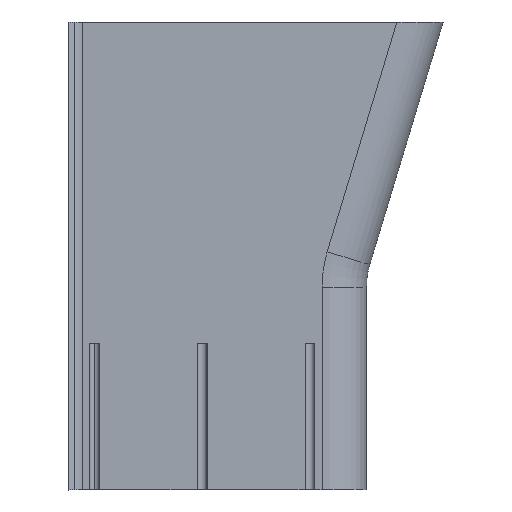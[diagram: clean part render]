
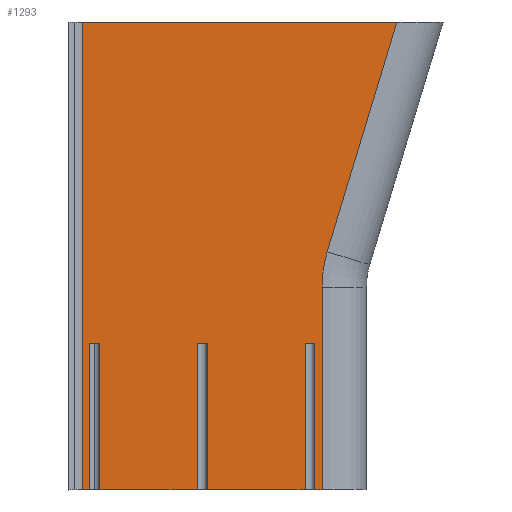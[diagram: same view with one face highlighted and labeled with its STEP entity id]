
A CAD part, left-side view. The second image highlights one B-rep face of the part: STEP entity #1293.
In plain terms, the highlighted planar face has unit normal (-1, 0, 0).
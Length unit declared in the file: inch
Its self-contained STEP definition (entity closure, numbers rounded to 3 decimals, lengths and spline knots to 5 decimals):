
#1 = VERTEX_POINT ( 'NONE', #1411 ) ;
#2 = DIRECTION ( 'NONE',  ( 0., -1., 0. ) ) ;
#8 = CARTESIAN_POINT ( 'NONE',  ( 4.52259, 2.87607, 6.34768 ) ) ;
#33 = CARTESIAN_POINT ( 'NONE',  ( 4.52259, 5.96984, 6.34768 ) ) ;
#66 = CARTESIAN_POINT ( 'NONE',  ( 4.52259, 4.9122, 1.57196 ) ) ;
#107 = VECTOR ( 'NONE', #1693, 39.37008 ) ;
#110 = VECTOR ( 'NONE', #1736, 39.37008 ) ;
#112 = LINE ( 'NONE', #1727, #110 ) ;
#113 = LINE ( 'NONE', #1715, #107 ) ;
#118 = LINE ( 'NONE', #1712, #127 ) ;
#127 = VECTOR ( 'NONE', #1710, 39.37008 ) ;
#130 = VECTOR ( 'NONE', #339, 39.37008 ) ;
#150 = VECTOR ( 'NONE', #289, 39.37008 ) ;
#156 = LINE ( 'NONE', #372, #150 ) ;
#160 = LINE ( 'NONE', #497, #130 ) ;
#168 = VECTOR ( 'NONE', #1691, 39.37008 ) ;
#169 = DIRECTION ( 'NONE',  ( 0., 1., 0. ) ) ;
#170 = VERTEX_POINT ( 'NONE', #1612 ) ;
#175 = LINE ( 'NONE', #1702, #168 ) ;
#179 = CARTESIAN_POINT ( 'NONE',  ( 4.52259, 3.63903, 1.57196 ) ) ;
#203 = LINE ( 'NONE', #685, #628 ) ;
#214 = CARTESIAN_POINT ( 'NONE',  ( 4.52259, 3.7122, 1.57196 ) ) ;
#216 = LINE ( 'NONE', #609, #410 ) ;
#231 = DIRECTION ( 'NONE',  ( 0., 1., 0. ) ) ;
#232 = CARTESIAN_POINT ( 'NONE',  ( 4.52259, 3.63903, 1.57196 ) ) ;
#237 = LINE ( 'NONE', #953, #244 ) ;
#244 = VECTOR ( 'NONE', #927, 39.37008 ) ;
#246 = DIRECTION ( 'NONE',  ( 0., 0., 1. ) ) ;
#255 = DIRECTION ( 'NONE',  ( -1., 0., 0. ) ) ;
#258 = CARTESIAN_POINT ( 'NONE',  ( 4.52259, 5.96984, 8.02732 ) ) ;
#272 = FACE_OUTER_BOUND ( 'NONE', #1458, .T. ) ;
#278 = PLANE ( 'NONE',  #649 ) ;
#289 = DIRECTION ( 'NONE',  ( 0., 0., -1. ) ) ;
#339 = DIRECTION ( 'NONE',  ( 0., 0., -1. ) ) ;
#365 = EDGE_CURVE ( 'NONE', #1374, #170, #786, .T. ) ;
#372 = CARTESIAN_POINT ( 'NONE',  ( 4.52259, 5.9122, 7.01889 ) ) ;
#410 = VECTOR ( 'NONE', #601, 39.37008 ) ;
#422 = CARTESIAN_POINT ( 'NONE',  ( 4.52259, 5.9122, 1.57196 ) ) ;
#423 = VECTOR ( 'NONE', #169, 39.37008 ) ;
#424 = LINE ( 'NONE', #179, #423 ) ;
#425 = DIRECTION ( 'NONE',  ( 0., 0., -1. ) ) ;
#427 = CARTESIAN_POINT ( 'NONE',  ( 4.52259, 4.8122, 7.01889 ) ) ;
#443 = VECTOR ( 'NONE', #1273, 39.37008 ) ;
#448 = LINE ( 'NONE', #232, #453 ) ;
#453 = VECTOR ( 'NONE', #231, 39.37008 ) ;
#490 = CARTESIAN_POINT ( 'NONE',  ( 4.52259, 6.0122, 1.57196 ) ) ;
#497 = CARTESIAN_POINT ( 'NONE',  ( 4.52259, 4.9122, 7.01889 ) ) ;
#515 = VERTEX_POINT ( 'NONE', #490 ) ;
#538 = DIRECTION ( 'NONE',  ( 0., 1., 0. ) ) ;
#539 = CARTESIAN_POINT ( 'NONE',  ( 4.52259, 3.63903, 1.57196 ) ) ;
#554 = LINE ( 'NONE', #427, #563 ) ;
#563 = VECTOR ( 'NONE', #425, 39.37008 ) ;
#570 = VERTEX_POINT ( 'NONE', #422 ) ;
#601 = DIRECTION ( 'NONE',  ( 0., 1., 0. ) ) ;
#608 = VECTOR ( 'NONE', #538, 39.37008 ) ;
#609 = CARTESIAN_POINT ( 'NONE',  ( 4.52259, 4.90544, 3.07196 ) ) ;
#610 = LINE ( 'NONE', #539, #608 ) ;
#628 = VECTOR ( 'NONE', #655, 39.37008 ) ;
#649 = AXIS2_PLACEMENT_3D ( 'NONE', #258, #255, #246 ) ;
#655 = DIRECTION ( 'NONE',  ( 0., 1., 0. ) ) ;
#668 = VECTOR ( 'NONE', #1101, 39.37008 ) ;
#673 = LINE ( 'NONE', #1129, #668 ) ;
#678 = VECTOR ( 'NONE', #1203, 39.37008 ) ;
#684 = LINE ( 'NONE', #1240, #678 ) ;
#685 = CARTESIAN_POINT ( 'NONE',  ( 4.52259, 3.63903, 1.57196 ) ) ;
#721 = DIRECTION ( 'NONE',  ( 0., 0., 1. ) ) ;
#724 = VECTOR ( 'NONE', #2, 39.37008 ) ;
#726 = EDGE_CURVE ( 'NONE', #1658, #1162, #727, .T. ) ;
#727 = LINE ( 'NONE', #33, #724 ) ;
#768 = DIRECTION ( 'NONE',  ( 1., 0., 0. ) ) ;
#786 = CIRCLE ( 'NONE', #884, 1.24053 ) ;
#805 = VERTEX_POINT ( 'NONE', #1672 ) ;
#808 = CARTESIAN_POINT ( 'NONE',  ( 4.52259, 2.3985, 3.64246 ) ) ;
#852 = VERTEX_POINT ( 'NONE', #1632 ) ;
#884 = AXIS2_PLACEMENT_3D ( 'NONE', #808, #768, #721 ) ;
#927 = DIRECTION ( 'NONE',  ( 0., 0., -1. ) ) ;
#941 = LINE ( 'NONE', #1333, #443 ) ;
#953 = CARTESIAN_POINT ( 'NONE',  ( 4.52259, 6.0122, 7.01889 ) ) ;
#989 = EDGE_CURVE ( 'NONE', #1, #1576, #684, .T. ) ;
#992 = VERTEX_POINT ( 'NONE', #1151 ) ;
#1013 = VERTEX_POINT ( 'NONE', #1133 ) ;
#1018 = EDGE_CURVE ( 'NONE', #1658, #1013, #673, .T. ) ;
#1055 = ORIENTED_EDGE ( 'NONE', *, *, #1419, .T. ) ;
#1083 = ORIENTED_EDGE ( 'NONE', *, *, #1412, .F. ) ;
#1088 = ORIENTED_EDGE ( 'NONE', *, *, #1300, .F. ) ;
#1092 = ORIENTED_EDGE ( 'NONE', *, *, #1246, .T. ) ;
#1094 = ORIENTED_EDGE ( 'NONE', *, *, #1441, .F. ) ;
#1097 = ORIENTED_EDGE ( 'NONE', *, *, #1322, .F. ) ;
#1098 = ORIENTED_EDGE ( 'NONE', *, *, #1018, .T. ) ;
#1101 = DIRECTION ( 'NONE',  ( 0., 0., -1. ) ) ;
#1126 = ORIENTED_EDGE ( 'NONE', *, *, #1706, .T. ) ;
#1129 = CARTESIAN_POINT ( 'NONE',  ( 4.52259, 6.08537, 8.02732 ) ) ;
#1133 = CARTESIAN_POINT ( 'NONE',  ( 4.52259, 6.08537, 1.57196 ) ) ;
#1151 = CARTESIAN_POINT ( 'NONE',  ( 4.52259, 6.0122, 3.07196 ) ) ;
#1161 = ORIENTED_EDGE ( 'NONE', *, *, #1400, .F. ) ;
#1162 = VERTEX_POINT ( 'NONE', #8 ) ;
#1185 = EDGE_CURVE ( 'NONE', #805, #1309, #203, .T. ) ;
#1203 = DIRECTION ( 'NONE',  ( 0., -1., 0. ) ) ;
#1223 = EDGE_CURVE ( 'NONE', #1556, #852, #610, .T. ) ;
#1240 = CARTESIAN_POINT ( 'NONE',  ( 4.52259, 4.90544, 3.07196 ) ) ;
#1246 = EDGE_CURVE ( 'NONE', #1549, #852, #554, .T. ) ;
#1273 = DIRECTION ( 'NONE',  ( 0., -1., 0. ) ) ;
#1293 = ADVANCED_FACE ( 'NONE', ( #272 ), #278, .T. ) ;
#1300 = EDGE_CURVE ( 'NONE', #1439, #570, #448, .T. ) ;
#1309 = VERTEX_POINT ( 'NONE', #214 ) ;
#1322 = EDGE_CURVE ( 'NONE', #515, #1013, #424, .T. ) ;
#1331 = ORIENTED_EDGE ( 'NONE', *, *, #1185, .F. ) ;
#1333 = CARTESIAN_POINT ( 'NONE',  ( 4.52259, 4.90544, 3.07196 ) ) ;
#1374 = VERTEX_POINT ( 'NONE', #1529 ) ;
#1400 = EDGE_CURVE ( 'NONE', #992, #515, #237, .T. ) ;
#1411 = CARTESIAN_POINT ( 'NONE',  ( 4.52259, 3.8122, 3.07196 ) ) ;
#1412 = EDGE_CURVE ( 'NONE', #1561, #992, #216, .T. ) ;
#1419 = EDGE_CURVE ( 'NONE', #1561, #570, #156, .T. ) ;
#1429 = CARTESIAN_POINT ( 'NONE',  ( 4.52259, 6.08537, 6.34768 ) ) ;
#1434 = CARTESIAN_POINT ( 'NONE',  ( 4.52259, 4.9122, 3.07196 ) ) ;
#1439 = VERTEX_POINT ( 'NONE', #66 ) ;
#1441 = EDGE_CURVE ( 'NONE', #1684, #1439, #160, .T. ) ;
#1458 = EDGE_LOOP ( 'NONE', ( #1517, #1098, #1097, #1161, #1083, #1055, #1088, #1094, #1126, #1092, #1531, #1671, #1575, #1642, #1331, #1648, #1590, #1475 ) ) ;
#1463 = EDGE_CURVE ( 'NONE', #1, #1556, #112, .T. ) ;
#1475 = ORIENTED_EDGE ( 'NONE', *, *, #1487, .T. ) ;
#1476 = EDGE_CURVE ( 'NONE', #1576, #1309, #118, .T. ) ;
#1484 = EDGE_CURVE ( 'NONE', #805, #1374, #113, .T. ) ;
#1487 = EDGE_CURVE ( 'NONE', #170, #1162, #175, .T. ) ;
#1516 = CARTESIAN_POINT ( 'NONE',  ( 4.52259, 3.7122, 3.07196 ) ) ;
#1517 = ORIENTED_EDGE ( 'NONE', *, *, #726, .F. ) ;
#1529 = CARTESIAN_POINT ( 'NONE',  ( 4.52259, 3.63903, 3.64246 ) ) ;
#1531 = ORIENTED_EDGE ( 'NONE', *, *, #1223, .F. ) ;
#1549 = VERTEX_POINT ( 'NONE', #1587 ) ;
#1556 = VERTEX_POINT ( 'NONE', #1595 ) ;
#1561 = VERTEX_POINT ( 'NONE', #1564 ) ;
#1564 = CARTESIAN_POINT ( 'NONE',  ( 4.52259, 5.9122, 3.07196 ) ) ;
#1575 = ORIENTED_EDGE ( 'NONE', *, *, #989, .T. ) ;
#1576 = VERTEX_POINT ( 'NONE', #1516 ) ;
#1587 = CARTESIAN_POINT ( 'NONE',  ( 4.52259, 4.8122, 3.07196 ) ) ;
#1590 = ORIENTED_EDGE ( 'NONE', *, *, #365, .T. ) ;
#1595 = CARTESIAN_POINT ( 'NONE',  ( 4.52259, 3.8122, 1.57196 ) ) ;
#1612 = CARTESIAN_POINT ( 'NONE',  ( 4.52259, 3.58587, 4.00171 ) ) ;
#1632 = CARTESIAN_POINT ( 'NONE',  ( 4.52259, 4.8122, 1.57196 ) ) ;
#1642 = ORIENTED_EDGE ( 'NONE', *, *, #1476, .T. ) ;
#1648 = ORIENTED_EDGE ( 'NONE', *, *, #1484, .T. ) ;
#1658 = VERTEX_POINT ( 'NONE', #1429 ) ;
#1671 = ORIENTED_EDGE ( 'NONE', *, *, #1463, .F. ) ;
#1672 = CARTESIAN_POINT ( 'NONE',  ( 4.52259, 3.63903, 1.57196 ) ) ;
#1684 = VERTEX_POINT ( 'NONE', #1434 ) ;
#1691 = DIRECTION ( 'NONE',  ( 0., -0.29, 0.957 ) ) ;
#1693 = DIRECTION ( 'NONE',  ( 0., 0., 1. ) ) ;
#1702 = CARTESIAN_POINT ( 'NONE',  ( 4.52259, 2.66996, 7.0289 ) ) ;
#1706 = EDGE_CURVE ( 'NONE', #1684, #1549, #941, .T. ) ;
#1710 = DIRECTION ( 'NONE',  ( 0., 0., -1. ) ) ;
#1712 = CARTESIAN_POINT ( 'NONE',  ( 4.52259, 3.7122, 7.01889 ) ) ;
#1715 = CARTESIAN_POINT ( 'NONE',  ( 4.52259, 3.63903, 8.02732 ) ) ;
#1727 = CARTESIAN_POINT ( 'NONE',  ( 4.52259, 3.8122, 7.01889 ) ) ;
#1736 = DIRECTION ( 'NONE',  ( 0., 0., -1. ) ) ;
